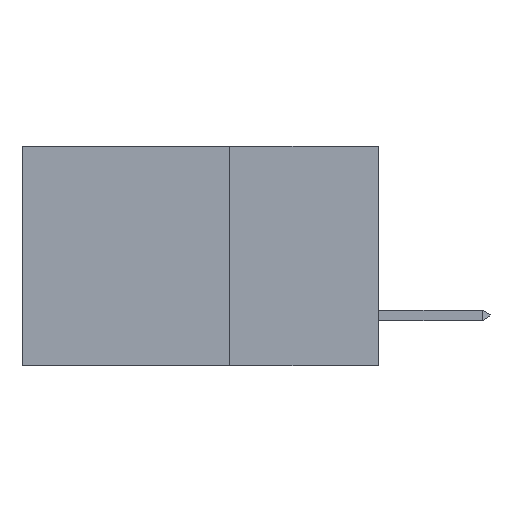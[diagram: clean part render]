
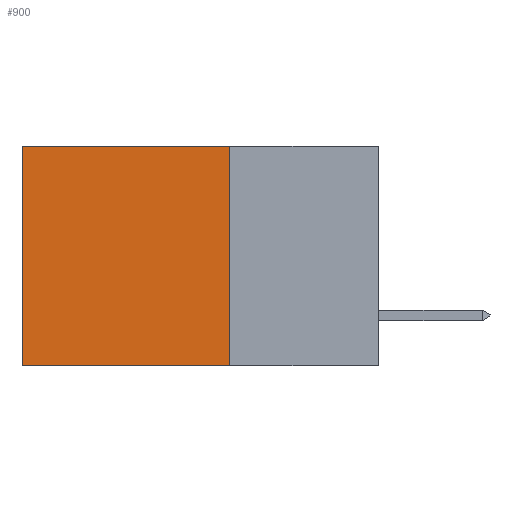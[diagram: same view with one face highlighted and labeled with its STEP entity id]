
A CAD part, left-side view. The second image highlights one B-rep face of the part: STEP entity #900.
In plain terms, the highlighted planar face has unit normal (-1, 0, 0).
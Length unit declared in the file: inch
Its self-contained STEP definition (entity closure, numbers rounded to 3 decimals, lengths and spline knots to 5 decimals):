
#97 = CARTESIAN_POINT ( 'NONE',  ( 0.2615, 0.6, -0.37 ) ) ;
#156 = EDGE_CURVE ( 'NONE', #12494, #8797, #908, .T. ) ;
#627 = CARTESIAN_POINT ( 'NONE',  ( 0.2615, 0.25, 0. ) ) ;
#846 = FACE_OUTER_BOUND ( 'NONE', #1141, .T. ) ;
#900 = ADVANCED_FACE ( 'NONE', ( #846 ), #15153, .F. ) ;
#908 = LINE ( 'NONE', #15208, #7255 ) ;
#991 = DIRECTION ( 'NONE',  ( 0., 1., 0. ) ) ;
#1141 = EDGE_LOOP ( 'NONE', ( #12304, #11481, #9999, #11182 ) ) ;
#2227 = LINE ( 'NONE', #11659, #14859 ) ;
#3080 = EDGE_CURVE ( 'NONE', #15049, #9446, #2227, .T. ) ;
#3733 = EDGE_CURVE ( 'NONE', #8797, #9446, #14481, .T. ) ;
#3859 = CARTESIAN_POINT ( 'NONE',  ( 0.2615, 0.25, -0.37 ) ) ;
#5464 = DIRECTION ( 'NONE',  ( 1., 0., 0. ) ) ;
#5515 = CARTESIAN_POINT ( 'NONE',  ( 0.2615, 0.25, -0.37 ) ) ;
#6046 = AXIS2_PLACEMENT_3D ( 'NONE', #12701, #5464, #10205 ) ;
#7002 = DIRECTION ( 'NONE',  ( 0., 0., -1. ) ) ;
#7255 = VECTOR ( 'NONE', #10492, 39.37008 ) ;
#7307 = VECTOR ( 'NONE', #991, 39.37008 ) ;
#7960 = LINE ( 'NONE', #12858, #7307 ) ;
#8458 = EDGE_CURVE ( 'NONE', #12494, #15049, #7960, .T. ) ;
#8797 = VERTEX_POINT ( 'NONE', #5515 ) ;
#9446 = VERTEX_POINT ( 'NONE', #97 ) ;
#9999 = ORIENTED_EDGE ( 'NONE', *, *, #156, .F. ) ;
#10092 = CARTESIAN_POINT ( 'NONE',  ( 0.2615, 0.6, 0. ) ) ;
#10205 = DIRECTION ( 'NONE',  ( 0., 0., -1. ) ) ;
#10492 = DIRECTION ( 'NONE',  ( 0., 0., -1. ) ) ;
#10795 = DIRECTION ( 'NONE',  ( 0., 1., 0. ) ) ;
#11182 = ORIENTED_EDGE ( 'NONE', *, *, #8458, .T. ) ;
#11481 = ORIENTED_EDGE ( 'NONE', *, *, #3733, .F. ) ;
#11659 = CARTESIAN_POINT ( 'NONE',  ( 0.2615, 0.6, -0.37 ) ) ;
#12304 = ORIENTED_EDGE ( 'NONE', *, *, #3080, .T. ) ;
#12494 = VERTEX_POINT ( 'NONE', #627 ) ;
#12701 = CARTESIAN_POINT ( 'NONE',  ( 0.2615, 0.25, -0.37 ) ) ;
#12858 = CARTESIAN_POINT ( 'NONE',  ( 0.2615, 0.25, 0. ) ) ;
#14481 = LINE ( 'NONE', #3859, #15386 ) ;
#14859 = VECTOR ( 'NONE', #7002, 39.37008 ) ;
#15049 = VERTEX_POINT ( 'NONE', #10092 ) ;
#15153 = PLANE ( 'NONE',  #6046 ) ;
#15208 = CARTESIAN_POINT ( 'NONE',  ( 0.2615, 0.25, -0.37 ) ) ;
#15386 = VECTOR ( 'NONE', #10795, 39.37008 ) ;
